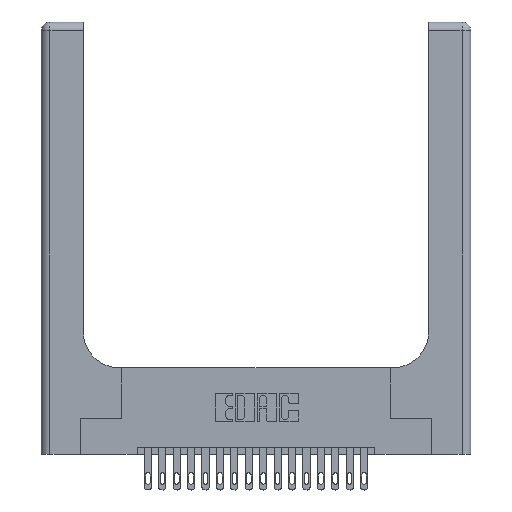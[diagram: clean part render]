
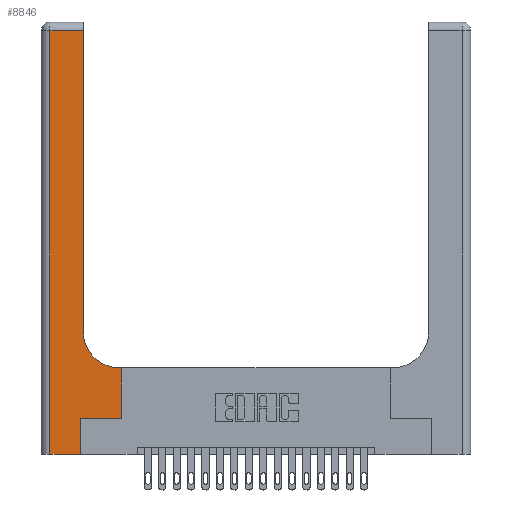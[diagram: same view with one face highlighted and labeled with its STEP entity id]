
A CAD part, top view. The second image highlights one B-rep face of the part: STEP entity #8846.
In plain terms, the highlighted planar face has unit normal (0, 0, 1).
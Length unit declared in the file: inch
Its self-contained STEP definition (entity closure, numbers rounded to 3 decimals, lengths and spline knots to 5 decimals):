
#185 = DIRECTION ( 'NONE',  ( 0., 0., -1. ) ) ;
#240 = DIRECTION ( 'NONE',  ( -1., 0., 0. ) ) ;
#293 = CARTESIAN_POINT ( 'NONE',  ( 0.269, 0.25, 0.37 ) ) ;
#797 = ORIENTED_EDGE ( 'NONE', *, *, #14310, .T. ) ;
#1524 = CARTESIAN_POINT ( 'NONE',  ( 0.5585, 0.25, 0.37 ) ) ;
#1781 = ORIENTED_EDGE ( 'NONE', *, *, #16758, .T. ) ;
#1955 = CARTESIAN_POINT ( 'NONE',  ( 0., 2.94, 0.37 ) ) ;
#2091 = AXIS2_PLACEMENT_3D ( 'NONE', #18166, #6592, #13324 ) ;
#2252 = LINE ( 'NONE', #15584, #10442 ) ;
#2308 = VERTEX_POINT ( 'NONE', #13312 ) ;
#2404 = CARTESIAN_POINT ( 'NONE',  ( 0.269, 0., 0.37 ) ) ;
#2668 = DIRECTION ( 'NONE',  ( -1., 0., 0. ) ) ;
#3085 = ORIENTED_EDGE ( 'NONE', *, *, #5414, .T. ) ;
#3379 = VERTEX_POINT ( 'NONE', #16600 ) ;
#3656 = CARTESIAN_POINT ( 'NONE',  ( 0.5415, 0.6, 0.37 ) ) ;
#3819 = VERTEX_POINT ( 'NONE', #3656 ) ;
#4101 = ORIENTED_EDGE ( 'NONE', *, *, #11389, .T. ) ;
#4560 = ORIENTED_EDGE ( 'NONE', *, *, #4891, .T. ) ;
#4891 = EDGE_CURVE ( 'NONE', #2308, #11145, #9715, .T. ) ;
#5262 = EDGE_CURVE ( 'NONE', #7933, #2308, #11210, .T. ) ;
#5414 = EDGE_CURVE ( 'NONE', #3379, #7933, #10186, .T. ) ;
#5856 = DIRECTION ( 'NONE',  ( 1., 0., 0. ) ) ;
#5937 = CIRCLE ( 'NONE', #2091, 0.25 ) ;
#5960 = VECTOR ( 'NONE', #8807, 39.37008 ) ;
#6592 = DIRECTION ( 'NONE',  ( 0., 0., -1. ) ) ;
#6700 = LINE ( 'NONE', #20530, #5960 ) ;
#6753 = DIRECTION ( 'NONE',  ( 1., 0., 0. ) ) ;
#7933 = VERTEX_POINT ( 'NONE', #10701 ) ;
#7971 = EDGE_CURVE ( 'NONE', #14058, #20272, #14914, .T. ) ;
#8807 = DIRECTION ( 'NONE',  ( 0., 1., 0. ) ) ;
#8846 = ADVANCED_FACE ( 'NONE', ( #10789 ), #11400, .F. ) ;
#9014 = DIRECTION ( 'NONE',  ( 0., 1., 0. ) ) ;
#9715 = LINE ( 'NONE', #10604, #17116 ) ;
#10186 = LINE ( 'NONE', #1955, #18383 ) ;
#10442 = VECTOR ( 'NONE', #2668, 39.37008 ) ;
#10491 = VECTOR ( 'NONE', #6753, 39.37008 ) ;
#10604 = CARTESIAN_POINT ( 'NONE',  ( 0., 0., 0.37 ) ) ;
#10701 = CARTESIAN_POINT ( 'NONE',  ( 0.06, 2.94, 0.37 ) ) ;
#10725 = LINE ( 'NONE', #17979, #10491 ) ;
#10772 = CARTESIAN_POINT ( 'NONE',  ( 0.5585, 0.25, 0.37 ) ) ;
#10789 = FACE_OUTER_BOUND ( 'NONE', #13115, .T. ) ;
#11145 = VERTEX_POINT ( 'NONE', #18254 ) ;
#11197 = VECTOR ( 'NONE', #13759, 39.37008 ) ;
#11210 = LINE ( 'NONE', #21001, #13743 ) ;
#11389 = EDGE_CURVE ( 'NONE', #15544, #3379, #6700, .T. ) ;
#11400 = PLANE ( 'NONE',  #20575 ) ;
#11519 = CARTESIAN_POINT ( 'NONE',  ( 0.5585, 0.6, 0.37 ) ) ;
#11697 = EDGE_CURVE ( 'NONE', #3819, #15544, #5937, .T. ) ;
#12038 = EDGE_CURVE ( 'NONE', #17196, #14058, #10725, .T. ) ;
#12418 = ORIENTED_EDGE ( 'NONE', *, *, #5262, .T. ) ;
#13115 = EDGE_LOOP ( 'NONE', ( #4101, #3085, #12418, #4560, #797, #17651, #21005, #1781, #20670 ) ) ;
#13312 = CARTESIAN_POINT ( 'NONE',  ( 0.06, 0., 0.37 ) ) ;
#13324 = DIRECTION ( 'NONE',  ( 1., 0., 0. ) ) ;
#13743 = VECTOR ( 'NONE', #21144, 39.37008 ) ;
#13759 = DIRECTION ( 'NONE',  ( 0., 1., 0. ) ) ;
#14058 = VERTEX_POINT ( 'NONE', #1524 ) ;
#14310 = EDGE_CURVE ( 'NONE', #11145, #17196, #14999, .T. ) ;
#14914 = LINE ( 'NONE', #10772, #17773 ) ;
#14999 = LINE ( 'NONE', #2404, #11197 ) ;
#15544 = VERTEX_POINT ( 'NONE', #15711 ) ;
#15584 = CARTESIAN_POINT ( 'NONE',  ( 0.2915, 0.6, 0.37 ) ) ;
#15711 = CARTESIAN_POINT ( 'NONE',  ( 0.2915, 0.85, 0.37 ) ) ;
#16600 = CARTESIAN_POINT ( 'NONE',  ( 0.2915, 2.94, 0.37 ) ) ;
#16758 = EDGE_CURVE ( 'NONE', #20272, #3819, #2252, .T. ) ;
#17116 = VECTOR ( 'NONE', #5856, 39.37008 ) ;
#17196 = VERTEX_POINT ( 'NONE', #293 ) ;
#17651 = ORIENTED_EDGE ( 'NONE', *, *, #12038, .T. ) ;
#17773 = VECTOR ( 'NONE', #9014, 39.37008 ) ;
#17979 = CARTESIAN_POINT ( 'NONE',  ( 0.269, 0.25, 0.37 ) ) ;
#18166 = CARTESIAN_POINT ( 'NONE',  ( 0.5415, 0.85, 0.37 ) ) ;
#18207 = CARTESIAN_POINT ( 'NONE',  ( 0., 3., 0.37 ) ) ;
#18254 = CARTESIAN_POINT ( 'NONE',  ( 0.269, 0., 0.37 ) ) ;
#18383 = VECTOR ( 'NONE', #240, 39.37008 ) ;
#19717 = DIRECTION ( 'NONE',  ( -1., 0., 0. ) ) ;
#20272 = VERTEX_POINT ( 'NONE', #11519 ) ;
#20530 = CARTESIAN_POINT ( 'NONE',  ( 0.2915, 3., 0.37 ) ) ;
#20575 = AXIS2_PLACEMENT_3D ( 'NONE', #18207, #185, #19717 ) ;
#20670 = ORIENTED_EDGE ( 'NONE', *, *, #11697, .T. ) ;
#21001 = CARTESIAN_POINT ( 'NONE',  ( 0.06, 3., 0.37 ) ) ;
#21005 = ORIENTED_EDGE ( 'NONE', *, *, #7971, .T. ) ;
#21144 = DIRECTION ( 'NONE',  ( 0., -1., 0. ) ) ;
